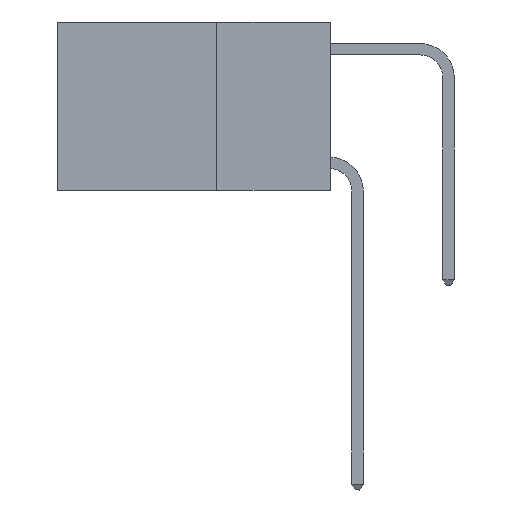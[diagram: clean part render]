
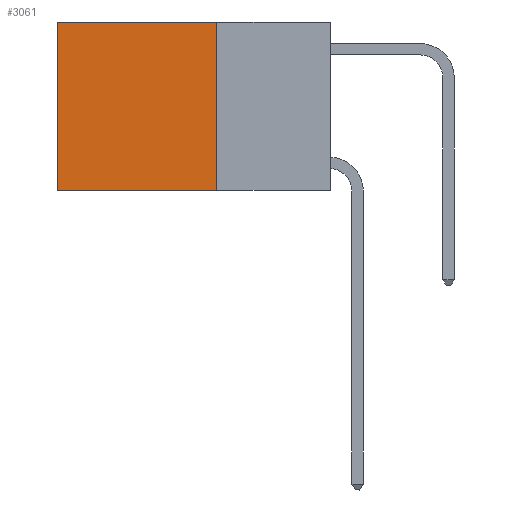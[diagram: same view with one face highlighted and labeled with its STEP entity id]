
A CAD part, left-side view. The second image highlights one B-rep face of the part: STEP entity #3061.
In plain terms, the highlighted planar face has unit normal (-1, 0, 0).
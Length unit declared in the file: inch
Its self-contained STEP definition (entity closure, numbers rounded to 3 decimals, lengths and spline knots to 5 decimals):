
#275 = EDGE_CURVE ( 'NONE', #7256, #16151, #8854, .T. ) ;
#521 = VECTOR ( 'NONE', #10554, 39.37008 ) ;
#929 = CARTESIAN_POINT ( 'NONE',  ( 0.2625, 0.6, -0.37 ) ) ;
#1265 = EDGE_CURVE ( 'NONE', #14833, #6670, #20564, .T. ) ;
#1581 = CARTESIAN_POINT ( 'NONE',  ( 0.2625, 0.25, 0. ) ) ;
#1980 = CARTESIAN_POINT ( 'NONE',  ( 0.2625, 0.25, -0.37 ) ) ;
#2829 = DIRECTION ( 'NONE',  ( 0., 0., -1. ) ) ;
#3061 = ADVANCED_FACE ( 'NONE', ( #20229 ), #21573, .F. ) ;
#6670 = VERTEX_POINT ( 'NONE', #15540 ) ;
#7256 = VERTEX_POINT ( 'NONE', #10283 ) ;
#8854 = LINE ( 'NONE', #1980, #19179 ) ;
#9079 = EDGE_LOOP ( 'NONE', ( #15756, #22380, #14905, #12642 ) ) ;
#9355 = AXIS2_PLACEMENT_3D ( 'NONE', #14139, #10573, #23412 ) ;
#10005 = LINE ( 'NONE', #11882, #18577 ) ;
#10194 = LINE ( 'NONE', #12386, #521 ) ;
#10283 = CARTESIAN_POINT ( 'NONE',  ( 0.2625, 0.25, -0.37 ) ) ;
#10554 = DIRECTION ( 'NONE',  ( 0., 0., -1. ) ) ;
#10573 = DIRECTION ( 'NONE',  ( 1., 0., 0. ) ) ;
#10782 = VECTOR ( 'NONE', #14286, 39.37008 ) ;
#11563 = EDGE_CURVE ( 'NONE', #6670, #16151, #10005, .T. ) ;
#11882 = CARTESIAN_POINT ( 'NONE',  ( 0.2625, 0.6, 0. ) ) ;
#12017 = CARTESIAN_POINT ( 'NONE',  ( 0.2625, 0.25, 0. ) ) ;
#12386 = CARTESIAN_POINT ( 'NONE',  ( 0.2625, 0.25, 0. ) ) ;
#12642 = ORIENTED_EDGE ( 'NONE', *, *, #1265, .T. ) ;
#14139 = CARTESIAN_POINT ( 'NONE',  ( 0.2625, 0.25, 0. ) ) ;
#14286 = DIRECTION ( 'NONE',  ( 0., 1., 0. ) ) ;
#14833 = VERTEX_POINT ( 'NONE', #12017 ) ;
#14905 = ORIENTED_EDGE ( 'NONE', *, *, #15624, .F. ) ;
#15540 = CARTESIAN_POINT ( 'NONE',  ( 0.2625, 0.6, 0. ) ) ;
#15624 = EDGE_CURVE ( 'NONE', #14833, #7256, #10194, .T. ) ;
#15756 = ORIENTED_EDGE ( 'NONE', *, *, #11563, .T. ) ;
#16151 = VERTEX_POINT ( 'NONE', #929 ) ;
#17216 = DIRECTION ( 'NONE',  ( 0., 1., 0. ) ) ;
#18577 = VECTOR ( 'NONE', #2829, 39.37008 ) ;
#19179 = VECTOR ( 'NONE', #17216, 39.37008 ) ;
#20229 = FACE_OUTER_BOUND ( 'NONE', #9079, .T. ) ;
#20564 = LINE ( 'NONE', #1581, #10782 ) ;
#21573 = PLANE ( 'NONE',  #9355 ) ;
#22380 = ORIENTED_EDGE ( 'NONE', *, *, #275, .F. ) ;
#23412 = DIRECTION ( 'NONE',  ( 0., 0., -1. ) ) ;
